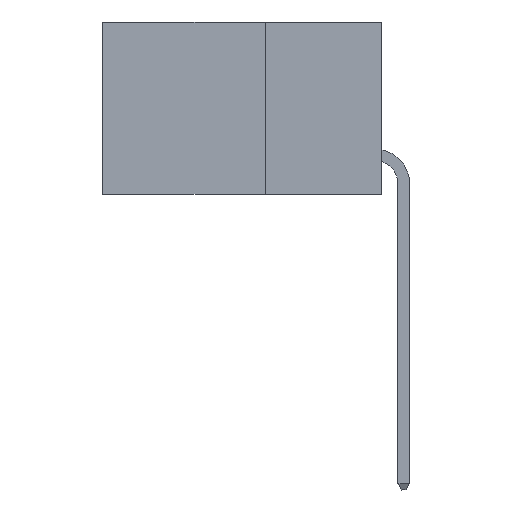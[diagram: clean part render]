
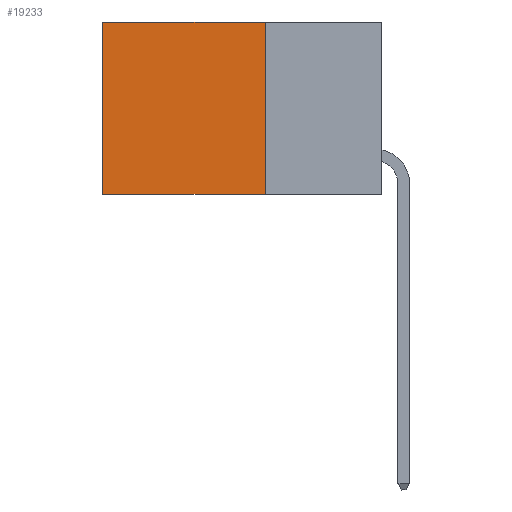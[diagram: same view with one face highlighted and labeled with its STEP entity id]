
A CAD part, left-side view. The second image highlights one B-rep face of the part: STEP entity #19233.
In plain terms, the highlighted planar face has unit normal (-1, 0, 0).
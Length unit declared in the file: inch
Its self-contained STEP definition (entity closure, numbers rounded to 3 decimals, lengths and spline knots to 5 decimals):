
#1634 = ORIENTED_EDGE ( 'NONE', *, *, #8942, .T. ) ;
#4356 = VERTEX_POINT ( 'NONE', #9014 ) ;
#5585 = EDGE_LOOP ( 'NONE', ( #1634, #12279, #7616, #23619 ) ) ;
#6519 = VECTOR ( 'NONE', #14885, 39.37008 ) ;
#7616 = ORIENTED_EDGE ( 'NONE', *, *, #25215, .F. ) ;
#8942 = EDGE_CURVE ( 'NONE', #27710, #4356, #21399, .T. ) ;
#9014 = CARTESIAN_POINT ( 'NONE',  ( 0.2875, 0.6, -0.37 ) ) ;
#9181 = CARTESIAN_POINT ( 'NONE',  ( 0.2875, 0.25, -0.37 ) ) ;
#9347 = VECTOR ( 'NONE', #21966, 39.37008 ) ;
#9436 = EDGE_CURVE ( 'NONE', #21462, #27710, #18533, .T. ) ;
#9596 = PLANE ( 'NONE',  #14999 ) ;
#9943 = CARTESIAN_POINT ( 'NONE',  ( 0.2875, 0.6, 0. ) ) ;
#11863 = CARTESIAN_POINT ( 'NONE',  ( 0.2875, 0.25, 0. ) ) ;
#12279 = ORIENTED_EDGE ( 'NONE', *, *, #23861, .F. ) ;
#12430 = CARTESIAN_POINT ( 'NONE',  ( 0.2875, 0.25, 0. ) ) ;
#13168 = VECTOR ( 'NONE', #21685, 39.37008 ) ;
#14117 = DIRECTION ( 'NONE',  ( 0., 0., -1. ) ) ;
#14885 = DIRECTION ( 'NONE',  ( 0., 1., 0. ) ) ;
#14999 = AXIS2_PLACEMENT_3D ( 'NONE', #11863, #27685, #14117 ) ;
#16869 = VECTOR ( 'NONE', #20474, 39.37008 ) ;
#17518 = CARTESIAN_POINT ( 'NONE',  ( 0.2875, 0.6, 0. ) ) ;
#18533 = LINE ( 'NONE', #26134, #6519 ) ;
#19233 = ADVANCED_FACE ( 'NONE', ( #24886 ), #9596, .F. ) ;
#19408 = CARTESIAN_POINT ( 'NONE',  ( 0.2875, 0.25, 0. ) ) ;
#20375 = CARTESIAN_POINT ( 'NONE',  ( 0.2875, 0.25, -0.37 ) ) ;
#20474 = DIRECTION ( 'NONE',  ( 0., 1., 0. ) ) ;
#21399 = LINE ( 'NONE', #17518, #9347 ) ;
#21462 = VERTEX_POINT ( 'NONE', #12430 ) ;
#21685 = DIRECTION ( 'NONE',  ( 0., 0., -1. ) ) ;
#21966 = DIRECTION ( 'NONE',  ( 0., 0., -1. ) ) ;
#23619 = ORIENTED_EDGE ( 'NONE', *, *, #9436, .T. ) ;
#23861 = EDGE_CURVE ( 'NONE', #27492, #4356, #27452, .T. ) ;
#24886 = FACE_OUTER_BOUND ( 'NONE', #5585, .T. ) ;
#25215 = EDGE_CURVE ( 'NONE', #21462, #27492, #25249, .T. ) ;
#25249 = LINE ( 'NONE', #19408, #13168 ) ;
#26134 = CARTESIAN_POINT ( 'NONE',  ( 0.2875, 0.25, 0. ) ) ;
#27452 = LINE ( 'NONE', #9181, #16869 ) ;
#27492 = VERTEX_POINT ( 'NONE', #20375 ) ;
#27685 = DIRECTION ( 'NONE',  ( 1., 0., 0. ) ) ;
#27710 = VERTEX_POINT ( 'NONE', #9943 ) ;
